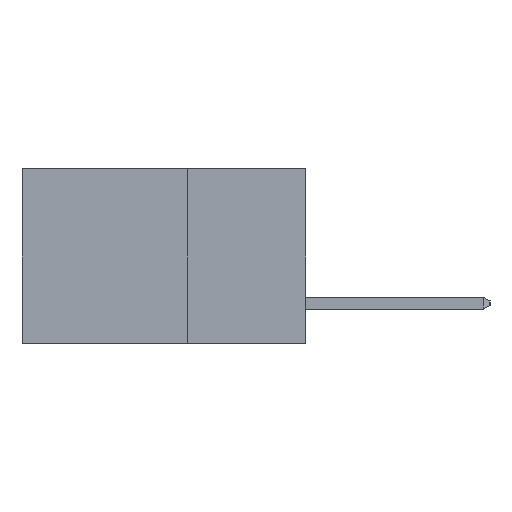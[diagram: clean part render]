
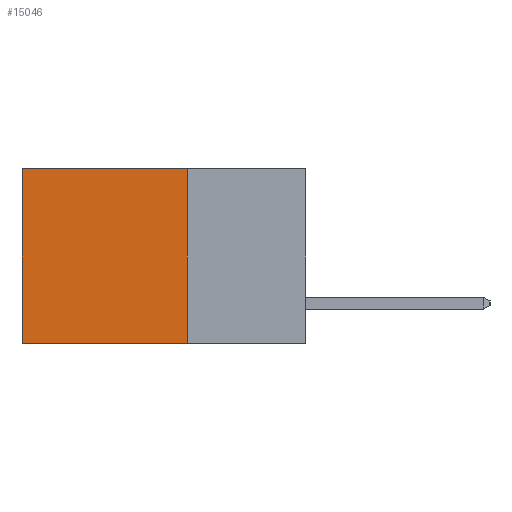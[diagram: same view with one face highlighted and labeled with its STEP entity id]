
A CAD part, left-side view. The second image highlights one B-rep face of the part: STEP entity #15046.
In plain terms, the highlighted planar face has unit normal (-1, 0, 0).
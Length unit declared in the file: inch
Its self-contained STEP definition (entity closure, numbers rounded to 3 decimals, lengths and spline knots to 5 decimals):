
#67 = CARTESIAN_POINT ( 'NONE',  ( 0.2615, 0.6, -0.37 ) ) ;
#1004 = VECTOR ( 'NONE', #18487, 39.37008 ) ;
#1139 = CARTESIAN_POINT ( 'NONE',  ( 0.2615, 0.25, 0. ) ) ;
#1159 = EDGE_CURVE ( 'NONE', #2845, #10505, #10800, .T. ) ;
#1522 = LINE ( 'NONE', #5451, #1004 ) ;
#2032 = LINE ( 'NONE', #15334, #18804 ) ;
#2216 = DIRECTION ( 'NONE',  ( 0., 1., 0. ) ) ;
#2376 = CARTESIAN_POINT ( 'NONE',  ( 0.2615, 0.25, -0.37 ) ) ;
#2845 = VERTEX_POINT ( 'NONE', #14035 ) ;
#3673 = PLANE ( 'NONE',  #7482 ) ;
#4105 = DIRECTION ( 'NONE',  ( 0., 1., 0. ) ) ;
#4815 = CARTESIAN_POINT ( 'NONE',  ( 0.2615, 0.6, -0.37 ) ) ;
#5451 = CARTESIAN_POINT ( 'NONE',  ( 0.2615, 0.25, -0.37 ) ) ;
#6245 = EDGE_CURVE ( 'NONE', #18739, #10505, #6275, .T. ) ;
#6275 = LINE ( 'NONE', #2376, #13934 ) ;
#6427 = VECTOR ( 'NONE', #11681, 39.37008 ) ;
#6920 = EDGE_LOOP ( 'NONE', ( #13989, #18308, #14820, #8967 ) ) ;
#7007 = CARTESIAN_POINT ( 'NONE',  ( 0.2615, 0.25, -0.37 ) ) ;
#7482 = AXIS2_PLACEMENT_3D ( 'NONE', #7007, #18365, #8621 ) ;
#8621 = DIRECTION ( 'NONE',  ( 0., 0., -1. ) ) ;
#8967 = ORIENTED_EDGE ( 'NONE', *, *, #18432, .T. ) ;
#10505 = VERTEX_POINT ( 'NONE', #4815 ) ;
#10800 = LINE ( 'NONE', #67, #6427 ) ;
#11681 = DIRECTION ( 'NONE',  ( 0., 0., -1. ) ) ;
#13934 = VECTOR ( 'NONE', #2216, 39.37008 ) ;
#13989 = ORIENTED_EDGE ( 'NONE', *, *, #1159, .T. ) ;
#14035 = CARTESIAN_POINT ( 'NONE',  ( 0.2615, 0.6, 0. ) ) ;
#14820 = ORIENTED_EDGE ( 'NONE', *, *, #18917, .F. ) ;
#15046 = ADVANCED_FACE ( 'NONE', ( #20446 ), #3673, .F. ) ;
#15334 = CARTESIAN_POINT ( 'NONE',  ( 0.2615, 0.25, 0. ) ) ;
#18022 = CARTESIAN_POINT ( 'NONE',  ( 0.2615, 0.25, -0.37 ) ) ;
#18308 = ORIENTED_EDGE ( 'NONE', *, *, #6245, .F. ) ;
#18365 = DIRECTION ( 'NONE',  ( 1., 0., 0. ) ) ;
#18432 = EDGE_CURVE ( 'NONE', #18546, #2845, #2032, .T. ) ;
#18487 = DIRECTION ( 'NONE',  ( 0., 0., -1. ) ) ;
#18546 = VERTEX_POINT ( 'NONE', #1139 ) ;
#18739 = VERTEX_POINT ( 'NONE', #18022 ) ;
#18804 = VECTOR ( 'NONE', #4105, 39.37008 ) ;
#18917 = EDGE_CURVE ( 'NONE', #18546, #18739, #1522, .T. ) ;
#20446 = FACE_OUTER_BOUND ( 'NONE', #6920, .T. ) ;
